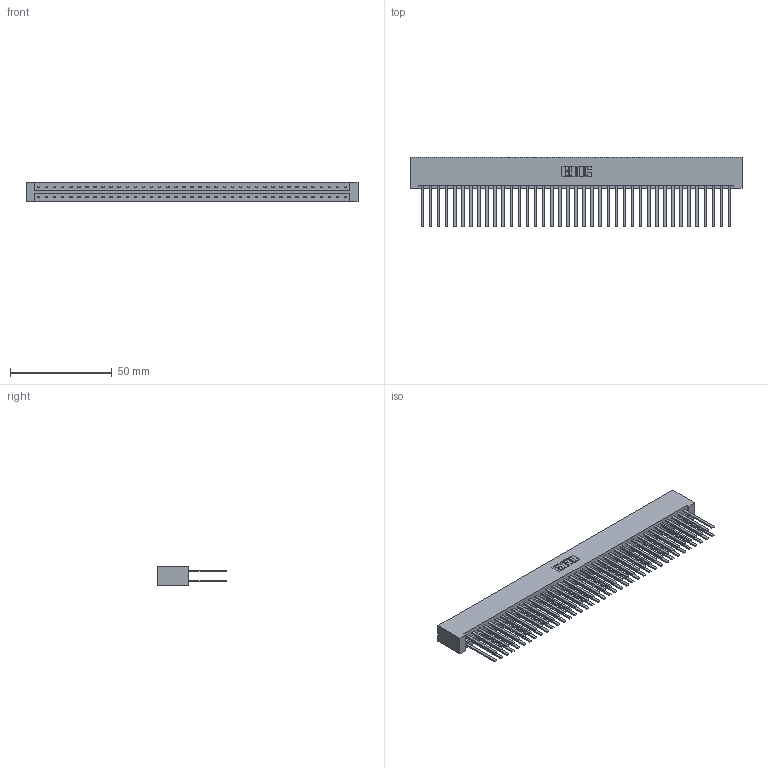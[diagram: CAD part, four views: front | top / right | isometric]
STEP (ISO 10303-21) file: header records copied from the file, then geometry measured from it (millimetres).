
FILE_DESCRIPTION (( 'STEP AP203' ), '1' );
FILE_NAME ('333-078-544-201.STEP', '2018-08-05T00:29:11', ( '' ), ( '' ), 'SwSTEP 2.0', 'SolidWorks 2016', '' );
FILE_SCHEMA (( 'CONFIG_CONTROL_DESIGN' ));
Length unit declared in the file: inch
Products named in the file (3): 333 Part_Lugless; 345-292-001_345-293-144; 333-078-544-201
Assembly tree (79 placements, depth 2):
  333-078-544-201
    333 Part_Lugless
    345-292-001_345-293-144  x78
Bounding box: 162.79 x 34.3 x 9.4 mm (x, y, z)
Volume: 18317.4 mm3; surface area: 25168.3 mm2
Topology: 79 solids, 79 shells, 3694 faces, 10973 edges, 7210 vertices
Faces by surface type: plane 2562, cylinder 1132
Entity records: 25017 total; most frequent: CARTESIAN_POINT 4146, ORIENTED_EDGE 4082, DIRECTION 3537, EDGE_CURVE 2041, VECTOR 1925, LINE 1925, VERTEX_POINT 1358, AXIS2_PLACEMENT_3D 806
